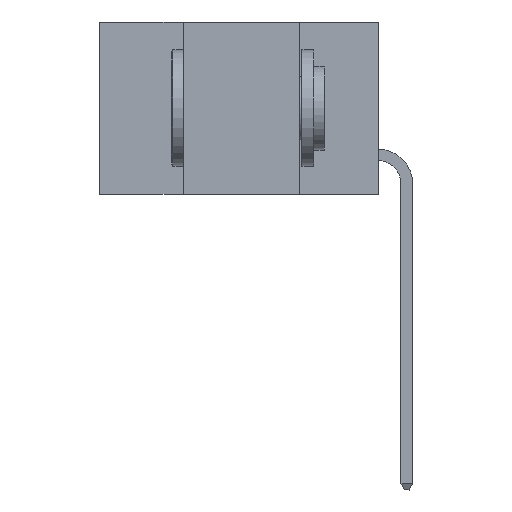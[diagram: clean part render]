
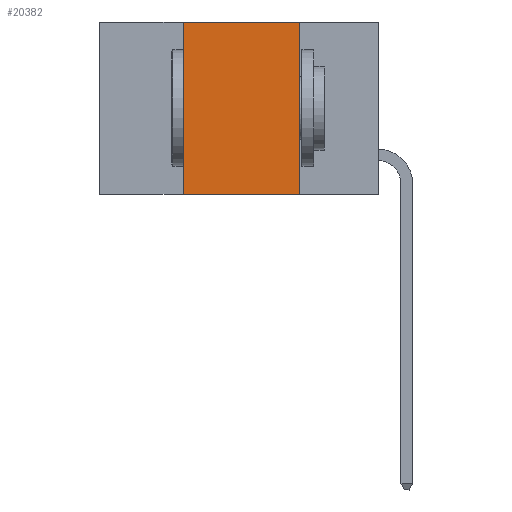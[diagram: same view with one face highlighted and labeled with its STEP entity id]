
A CAD part, left-side view. The second image highlights one B-rep face of the part: STEP entity #20382.
In plain terms, the highlighted planar face has unit normal (-1, 0, 0).
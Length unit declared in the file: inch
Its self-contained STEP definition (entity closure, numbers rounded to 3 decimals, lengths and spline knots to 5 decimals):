
#9 = DIRECTION ( 'NONE',  ( 0., 0., -1. ) ) ;
#126 = VECTOR ( 'NONE', #11825, 39.37008 ) ;
#774 = EDGE_CURVE ( 'NONE', #22635, #6698, #9273, .T. ) ;
#1699 = VERTEX_POINT ( 'NONE', #12467 ) ;
#2987 = FACE_OUTER_BOUND ( 'NONE', #21827, .T. ) ;
#3876 = VECTOR ( 'NONE', #18719, 39.37008 ) ;
#3907 = CARTESIAN_POINT ( 'NONE',  ( 0., 0.17, 0. ) ) ;
#4674 = CARTESIAN_POINT ( 'NONE',  ( 0., 0.6, -0.37 ) ) ;
#4868 = EDGE_CURVE ( 'NONE', #19180, #6698, #19106, .T. ) ;
#6698 = VERTEX_POINT ( 'NONE', #8177 ) ;
#7739 = VECTOR ( 'NONE', #10670, 39.37008 ) ;
#8109 = ORIENTED_EDGE ( 'NONE', *, *, #4868, .T. ) ;
#8177 = CARTESIAN_POINT ( 'NONE',  ( 0., 0.17, -0.37 ) ) ;
#8517 = CARTESIAN_POINT ( 'NONE',  ( 0., 0.42, 0. ) ) ;
#9156 = PLANE ( 'NONE',  #19822 ) ;
#9273 = LINE ( 'NONE', #3907, #3876 ) ;
#9745 = CARTESIAN_POINT ( 'NONE',  ( 0., 0.17, 0. ) ) ;
#10064 = ORIENTED_EDGE ( 'NONE', *, *, #21942, .F. ) ;
#10670 = DIRECTION ( 'NONE',  ( 0., -1., 0. ) ) ;
#10943 = DIRECTION ( 'NONE',  ( 1., 0., 0. ) ) ;
#11675 = VECTOR ( 'NONE', #17245, 39.37008 ) ;
#11825 = DIRECTION ( 'NONE',  ( 0., -1., 0. ) ) ;
#12467 = CARTESIAN_POINT ( 'NONE',  ( 0., 0.42, 0. ) ) ;
#13704 = ORIENTED_EDGE ( 'NONE', *, *, #774, .F. ) ;
#16364 = LINE ( 'NONE', #8517, #11675 ) ;
#17245 = DIRECTION ( 'NONE',  ( 0., 0., 1. ) ) ;
#18719 = DIRECTION ( 'NONE',  ( 0., 0., -1. ) ) ;
#19106 = LINE ( 'NONE', #4674, #126 ) ;
#19180 = VERTEX_POINT ( 'NONE', #22742 ) ;
#19317 = CARTESIAN_POINT ( 'NONE',  ( 0., 0.6, 0. ) ) ;
#19822 = AXIS2_PLACEMENT_3D ( 'NONE', #21280, #10943, #9 ) ;
#20382 = ADVANCED_FACE ( 'NONE', ( #2987 ), #9156, .F. ) ;
#20889 = ORIENTED_EDGE ( 'NONE', *, *, #21392, .F. ) ;
#21280 = CARTESIAN_POINT ( 'NONE',  ( 0., 0.6, 0. ) ) ;
#21392 = EDGE_CURVE ( 'NONE', #19180, #1699, #16364, .T. ) ;
#21827 = EDGE_LOOP ( 'NONE', ( #13704, #10064, #20889, #8109 ) ) ;
#21942 = EDGE_CURVE ( 'NONE', #1699, #22635, #22112, .T. ) ;
#22112 = LINE ( 'NONE', #19317, #7739 ) ;
#22635 = VERTEX_POINT ( 'NONE', #9745 ) ;
#22742 = CARTESIAN_POINT ( 'NONE',  ( 0., 0.42, -0.37 ) ) ;
